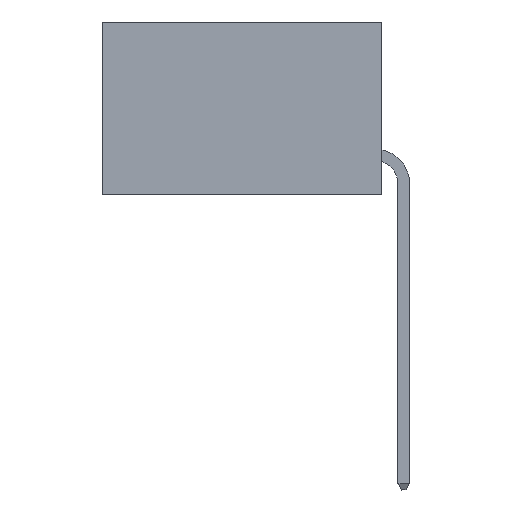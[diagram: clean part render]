
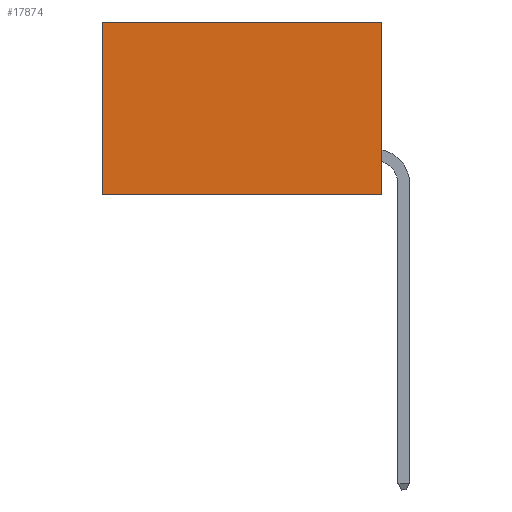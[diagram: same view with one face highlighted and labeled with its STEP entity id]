
A CAD part, left-side view. The second image highlights one B-rep face of the part: STEP entity #17874.
In plain terms, the highlighted planar face has unit normal (-1, 0, 0).
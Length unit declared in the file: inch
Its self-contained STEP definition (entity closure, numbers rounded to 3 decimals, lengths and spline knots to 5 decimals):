
#577 = VERTEX_POINT ( 'NONE', #11613 ) ;
#1805 = EDGE_CURVE ( 'NONE', #2565, #40471, #27677, .T. ) ;
#2565 = VERTEX_POINT ( 'NONE', #39057 ) ;
#3146 = DIRECTION ( 'NONE',  ( 0., 1., 0. ) ) ;
#6163 = CARTESIAN_POINT ( 'NONE',  ( 0.2875, 0., 0. ) ) ;
#9167 = ORIENTED_EDGE ( 'NONE', *, *, #11490, .T. ) ;
#9379 = PLANE ( 'NONE',  #33765 ) ;
#10866 = CARTESIAN_POINT ( 'NONE',  ( 0.2875, 0., -0.37 ) ) ;
#11009 = VECTOR ( 'NONE', #28574, 39.37008 ) ;
#11249 = CARTESIAN_POINT ( 'NONE',  ( 0.2875, 0., 0. ) ) ;
#11490 = EDGE_CURVE ( 'NONE', #577, #17974, #16714, .T. ) ;
#11520 = VECTOR ( 'NONE', #3146, 39.37008 ) ;
#11613 = CARTESIAN_POINT ( 'NONE',  ( 0.2875, 0., 0. ) ) ;
#11849 = ORIENTED_EDGE ( 'NONE', *, *, #39289, .T. ) ;
#16714 = LINE ( 'NONE', #18736, #11009 ) ;
#17874 = ADVANCED_FACE ( 'NONE', ( #24821 ), #9379, .F. ) ;
#17974 = VERTEX_POINT ( 'NONE', #33575 ) ;
#18736 = CARTESIAN_POINT ( 'NONE',  ( 0.2875, 0., 0. ) ) ;
#21046 = DIRECTION ( 'NONE',  ( 0., 0., -1. ) ) ;
#24821 = FACE_OUTER_BOUND ( 'NONE', #35193, .T. ) ;
#26722 = LINE ( 'NONE', #11249, #28313 ) ;
#27481 = CARTESIAN_POINT ( 'NONE',  ( 0.2875, 0.6, 0. ) ) ;
#27677 = LINE ( 'NONE', #10866, #11520 ) ;
#28313 = VECTOR ( 'NONE', #31552, 39.37008 ) ;
#28513 = CARTESIAN_POINT ( 'NONE',  ( 0.2875, 0.6, -0.37 ) ) ;
#28574 = DIRECTION ( 'NONE',  ( 0., 1., 0. ) ) ;
#29219 = DIRECTION ( 'NONE',  ( 1., 0., 0. ) ) ;
#31552 = DIRECTION ( 'NONE',  ( 0., 0., -1. ) ) ;
#31569 = EDGE_CURVE ( 'NONE', #577, #2565, #26722, .T. ) ;
#32754 = DIRECTION ( 'NONE',  ( 0., 0., -1. ) ) ;
#33575 = CARTESIAN_POINT ( 'NONE',  ( 0.2875, 0.6, 0. ) ) ;
#33765 = AXIS2_PLACEMENT_3D ( 'NONE', #6163, #29219, #32754 ) ;
#33988 = VECTOR ( 'NONE', #21046, 39.37008 ) ;
#35193 = EDGE_LOOP ( 'NONE', ( #11849, #37179, #36081, #9167 ) ) ;
#36081 = ORIENTED_EDGE ( 'NONE', *, *, #31569, .F. ) ;
#36600 = LINE ( 'NONE', #27481, #33988 ) ;
#37179 = ORIENTED_EDGE ( 'NONE', *, *, #1805, .F. ) ;
#39057 = CARTESIAN_POINT ( 'NONE',  ( 0.2875, 0., -0.37 ) ) ;
#39289 = EDGE_CURVE ( 'NONE', #17974, #40471, #36600, .T. ) ;
#40471 = VERTEX_POINT ( 'NONE', #28513 ) ;
